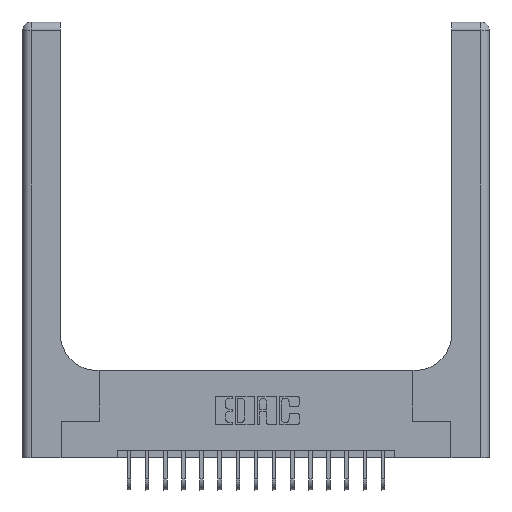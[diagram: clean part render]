
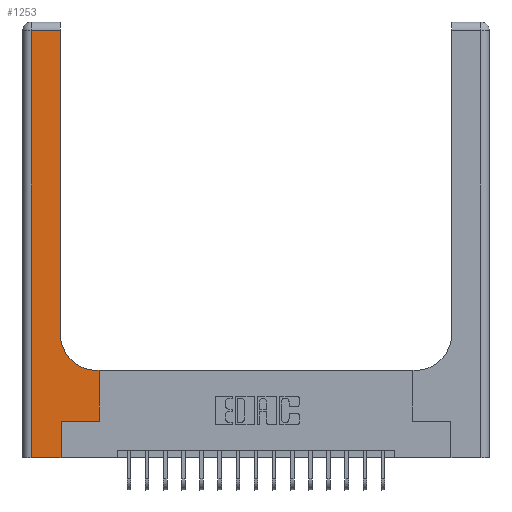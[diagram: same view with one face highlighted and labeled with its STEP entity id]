
A CAD part, top view. The second image highlights one B-rep face of the part: STEP entity #1253.
In plain terms, the highlighted planar face has unit normal (0, 0, 1).
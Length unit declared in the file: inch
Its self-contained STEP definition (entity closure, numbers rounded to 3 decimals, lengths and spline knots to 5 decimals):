
#264 = ORIENTED_EDGE ( 'NONE', *, *, #4306, .T. ) ;
#447 = EDGE_CURVE ( 'NONE', #16676, #17118, #3067, .T. ) ;
#712 = PLANE ( 'NONE',  #7972 ) ;
#768 = VECTOR ( 'NONE', #4629, 39.37008 ) ;
#1167 = ORIENTED_EDGE ( 'NONE', *, *, #9886, .T. ) ;
#1253 = ADVANCED_FACE ( 'NONE', ( #8836 ), #712, .F. ) ;
#1374 = LINE ( 'NONE', #12652, #768 ) ;
#1505 = DIRECTION ( 'NONE',  ( 0., 1., 0. ) ) ;
#1861 = VERTEX_POINT ( 'NONE', #14259 ) ;
#1981 = ORIENTED_EDGE ( 'NONE', *, *, #16889, .T. ) ;
#2421 = CIRCLE ( 'NONE', #16228, 0.25 ) ;
#2482 = CARTESIAN_POINT ( 'NONE',  ( 0., 3., 0.37 ) ) ;
#2739 = CARTESIAN_POINT ( 'NONE',  ( 0.06, 3., 0.37 ) ) ;
#2910 = CARTESIAN_POINT ( 'NONE',  ( 0.51, 0.85, 0.37 ) ) ;
#3067 = LINE ( 'NONE', #2739, #9568 ) ;
#3071 = DIRECTION ( 'NONE',  ( -1., 0., 0. ) ) ;
#3120 = CARTESIAN_POINT ( 'NONE',  ( 0.265, 0., 0.37 ) ) ;
#3309 = LINE ( 'NONE', #9757, #6482 ) ;
#3739 = VERTEX_POINT ( 'NONE', #10870 ) ;
#4306 = EDGE_CURVE ( 'NONE', #15947, #16676, #14366, .T. ) ;
#4333 = VECTOR ( 'NONE', #3071, 39.37008 ) ;
#4629 = DIRECTION ( 'NONE',  ( 1., 0., 0. ) ) ;
#4717 = ORIENTED_EDGE ( 'NONE', *, *, #16559, .T. ) ;
#5549 = DIRECTION ( 'NONE',  ( 0., 0., -1. ) ) ;
#6213 = DIRECTION ( 'NONE',  ( 0., -1., 0. ) ) ;
#6307 = VECTOR ( 'NONE', #8698, 39.37008 ) ;
#6450 = CARTESIAN_POINT ( 'NONE',  ( 0.528, 0.25, 0.37 ) ) ;
#6482 = VECTOR ( 'NONE', #19247, 39.37008 ) ;
#6491 = VERTEX_POINT ( 'NONE', #3120 ) ;
#6619 = EDGE_CURVE ( 'NONE', #6491, #9097, #10282, .T. ) ;
#6953 = CARTESIAN_POINT ( 'NONE',  ( 0.26, 3., 0.37 ) ) ;
#7497 = CARTESIAN_POINT ( 'NONE',  ( 0.265, 0., 0.37 ) ) ;
#7661 = EDGE_LOOP ( 'NONE', ( #18403, #264, #8628, #4717, #16700, #1981, #1167, #10905, #16571 ) ) ;
#7972 = AXIS2_PLACEMENT_3D ( 'NONE', #2482, #5549, #15255 ) ;
#8053 = CARTESIAN_POINT ( 'NONE',  ( 0., 2.94, 0.37 ) ) ;
#8628 = ORIENTED_EDGE ( 'NONE', *, *, #447, .T. ) ;
#8698 = DIRECTION ( 'NONE',  ( 0., 1., 0. ) ) ;
#8836 = FACE_OUTER_BOUND ( 'NONE', #7661, .T. ) ;
#9097 = VERTEX_POINT ( 'NONE', #10350 ) ;
#9248 = DIRECTION ( 'NONE',  ( 0., 0., -1. ) ) ;
#9568 = VECTOR ( 'NONE', #6213, 39.37008 ) ;
#9757 = CARTESIAN_POINT ( 'NONE',  ( 0., 0., 0.37 ) ) ;
#9886 = EDGE_CURVE ( 'NONE', #1861, #14771, #20710, .T. ) ;
#10282 = LINE ( 'NONE', #7497, #6307 ) ;
#10317 = VECTOR ( 'NONE', #19346, 39.37008 ) ;
#10321 = CARTESIAN_POINT ( 'NONE',  ( 0.06, 0., 0.37 ) ) ;
#10350 = CARTESIAN_POINT ( 'NONE',  ( 0.265, 0.25, 0.37 ) ) ;
#10395 = EDGE_CURVE ( 'NONE', #14771, #3739, #11197, .T. ) ;
#10870 = CARTESIAN_POINT ( 'NONE',  ( 0.51, 0.6, 0.37 ) ) ;
#10905 = ORIENTED_EDGE ( 'NONE', *, *, #10395, .T. ) ;
#11077 = VECTOR ( 'NONE', #1505, 39.37008 ) ;
#11127 = CARTESIAN_POINT ( 'NONE',  ( 0.26, 2.94, 0.37 ) ) ;
#11197 = LINE ( 'NONE', #14548, #4333 ) ;
#12190 = VERTEX_POINT ( 'NONE', #18529 ) ;
#12652 = CARTESIAN_POINT ( 'NONE',  ( 0.265, 0.25, 0.37 ) ) ;
#14259 = CARTESIAN_POINT ( 'NONE',  ( 0.528, 0.25, 0.37 ) ) ;
#14366 = LINE ( 'NONE', #8053, #10317 ) ;
#14548 = CARTESIAN_POINT ( 'NONE',  ( 0.26, 0.6, 0.37 ) ) ;
#14771 = VERTEX_POINT ( 'NONE', #15071 ) ;
#14995 = CARTESIAN_POINT ( 'NONE',  ( 0.06, 2.94, 0.37 ) ) ;
#15071 = CARTESIAN_POINT ( 'NONE',  ( 0.528, 0.6, 0.37 ) ) ;
#15255 = DIRECTION ( 'NONE',  ( -1., 0., 0. ) ) ;
#15277 = LINE ( 'NONE', #6953, #19685 ) ;
#15378 = EDGE_CURVE ( 'NONE', #3739, #12190, #2421, .T. ) ;
#15947 = VERTEX_POINT ( 'NONE', #11127 ) ;
#16228 = AXIS2_PLACEMENT_3D ( 'NONE', #2910, #9248, #17367 ) ;
#16559 = EDGE_CURVE ( 'NONE', #17118, #6491, #3309, .T. ) ;
#16571 = ORIENTED_EDGE ( 'NONE', *, *, #15378, .T. ) ;
#16676 = VERTEX_POINT ( 'NONE', #14995 ) ;
#16700 = ORIENTED_EDGE ( 'NONE', *, *, #6619, .T. ) ;
#16754 = DIRECTION ( 'NONE',  ( 0., 1., 0. ) ) ;
#16889 = EDGE_CURVE ( 'NONE', #9097, #1861, #1374, .T. ) ;
#17118 = VERTEX_POINT ( 'NONE', #10321 ) ;
#17367 = DIRECTION ( 'NONE',  ( 1., 0., 0. ) ) ;
#18403 = ORIENTED_EDGE ( 'NONE', *, *, #19658, .T. ) ;
#18529 = CARTESIAN_POINT ( 'NONE',  ( 0.26, 0.85, 0.37 ) ) ;
#19247 = DIRECTION ( 'NONE',  ( 1., 0., 0. ) ) ;
#19346 = DIRECTION ( 'NONE',  ( -1., 0., 0. ) ) ;
#19658 = EDGE_CURVE ( 'NONE', #12190, #15947, #15277, .T. ) ;
#19685 = VECTOR ( 'NONE', #16754, 39.37008 ) ;
#20710 = LINE ( 'NONE', #6450, #11077 ) ;
